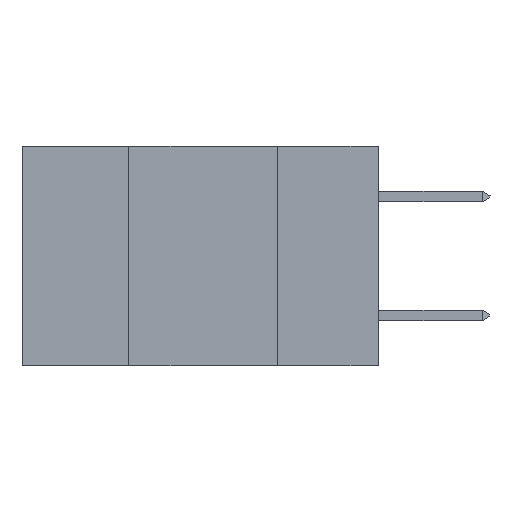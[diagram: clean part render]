
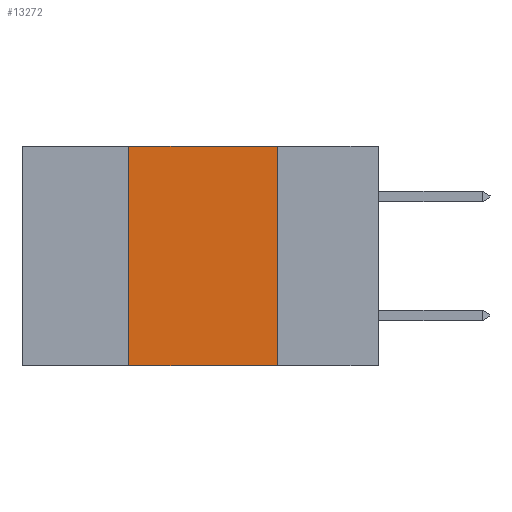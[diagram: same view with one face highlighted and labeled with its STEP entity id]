
A CAD part, left-side view. The second image highlights one B-rep face of the part: STEP entity #13272.
In plain terms, the highlighted planar face has unit normal (-1, 0, 0).
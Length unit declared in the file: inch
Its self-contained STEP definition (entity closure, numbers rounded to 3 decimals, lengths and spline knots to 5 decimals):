
#197 = CARTESIAN_POINT ( 'NONE',  ( 0., 0.6, 0. ) ) ;
#350 = ORIENTED_EDGE ( 'NONE', *, *, #10341, .F. ) ;
#1192 = DIRECTION ( 'NONE',  ( 0., 0., 1. ) ) ;
#1519 = CARTESIAN_POINT ( 'NONE',  ( 0., 0.6, 0. ) ) ;
#1670 = CARTESIAN_POINT ( 'NONE',  ( 0., 0.42, -0.37 ) ) ;
#1998 = VERTEX_POINT ( 'NONE', #1670 ) ;
#2620 = VERTEX_POINT ( 'NONE', #10498 ) ;
#3297 = EDGE_CURVE ( 'NONE', #14673, #6097, #5905, .T. ) ;
#4455 = ORIENTED_EDGE ( 'NONE', *, *, #9781, .T. ) ;
#4485 = LINE ( 'NONE', #14701, #12898 ) ;
#4685 = CARTESIAN_POINT ( 'NONE',  ( 0., 0.42, -0.37 ) ) ;
#5021 = PLANE ( 'NONE',  #14665 ) ;
#5244 = DIRECTION ( 'NONE',  ( 0., 0., -1. ) ) ;
#5829 = CARTESIAN_POINT ( 'NONE',  ( 0., 0.17, -0.37 ) ) ;
#5905 = LINE ( 'NONE', #5829, #13860 ) ;
#6097 = VERTEX_POINT ( 'NONE', #14509 ) ;
#7377 = VECTOR ( 'NONE', #1192, 39.37008 ) ;
#7645 = ORIENTED_EDGE ( 'NONE', *, *, #3297, .F. ) ;
#8090 = ORIENTED_EDGE ( 'NONE', *, *, #10408, .F. ) ;
#8344 = DIRECTION ( 'NONE',  ( 1., 0., 0. ) ) ;
#9451 = DIRECTION ( 'NONE',  ( 0., -1., 0. ) ) ;
#9781 = EDGE_CURVE ( 'NONE', #1998, #6097, #4485, .T. ) ;
#10341 = EDGE_CURVE ( 'NONE', #1998, #2620, #12700, .T. ) ;
#10408 = EDGE_CURVE ( 'NONE', #2620, #14673, #10438, .T. ) ;
#10438 = LINE ( 'NONE', #197, #10762 ) ;
#10498 = CARTESIAN_POINT ( 'NONE',  ( 0., 0.42, 0. ) ) ;
#10762 = VECTOR ( 'NONE', #9451, 39.37008 ) ;
#11295 = DIRECTION ( 'NONE',  ( 0., -1., 0. ) ) ;
#12700 = LINE ( 'NONE', #4685, #7377 ) ;
#12898 = VECTOR ( 'NONE', #11295, 39.37008 ) ;
#13272 = ADVANCED_FACE ( 'NONE', ( #14252 ), #5021, .F. ) ;
#13312 = EDGE_LOOP ( 'NONE', ( #7645, #8090, #350, #4455 ) ) ;
#13689 = DIRECTION ( 'NONE',  ( 0., 0., -1. ) ) ;
#13860 = VECTOR ( 'NONE', #13689, 39.37008 ) ;
#14252 = FACE_OUTER_BOUND ( 'NONE', #13312, .T. ) ;
#14509 = CARTESIAN_POINT ( 'NONE',  ( 0., 0.17, -0.37 ) ) ;
#14665 = AXIS2_PLACEMENT_3D ( 'NONE', #1519, #8344, #5244 ) ;
#14673 = VERTEX_POINT ( 'NONE', #14889 ) ;
#14701 = CARTESIAN_POINT ( 'NONE',  ( 0., 0.6, -0.37 ) ) ;
#14889 = CARTESIAN_POINT ( 'NONE',  ( 0., 0.17, 0. ) ) ;
